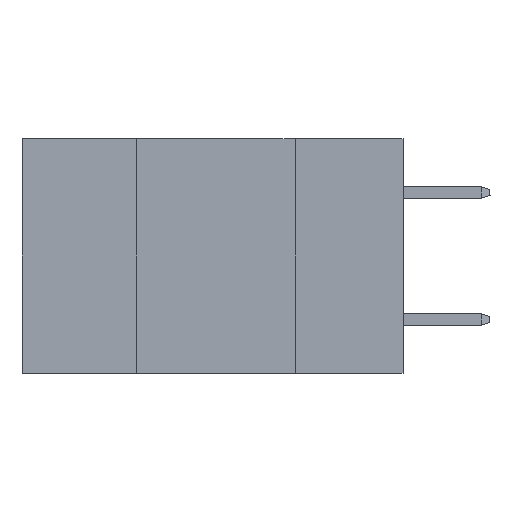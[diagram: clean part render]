
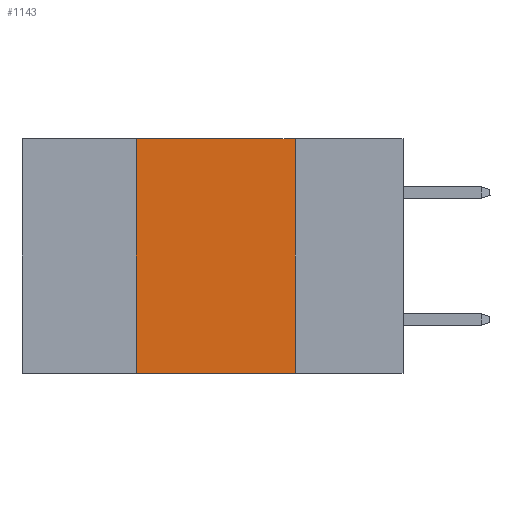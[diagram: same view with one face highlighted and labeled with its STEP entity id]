
A CAD part, left-side view. The second image highlights one B-rep face of the part: STEP entity #1143.
In plain terms, the highlighted planar face has unit normal (-1, 0, 0).
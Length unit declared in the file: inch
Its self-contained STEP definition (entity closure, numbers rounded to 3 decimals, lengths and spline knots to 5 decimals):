
#374 = VERTEX_POINT ( 'NONE', #19718 ) ;
#496 = CARTESIAN_POINT ( 'NONE',  ( 0., 0.17, 0. ) ) ;
#780 = LINE ( 'NONE', #14381, #11953 ) ;
#810 = LINE ( 'NONE', #7644, #19834 ) ;
#1143 = ADVANCED_FACE ( 'NONE', ( #3418 ), #10226, .F. ) ;
#1242 = LINE ( 'NONE', #496, #16465 ) ;
#2068 = DIRECTION ( 'NONE',  ( 1., 0., 0. ) ) ;
#2464 = DIRECTION ( 'NONE',  ( 0., -1., 0. ) ) ;
#3418 = FACE_OUTER_BOUND ( 'NONE', #9105, .T. ) ;
#4226 = LINE ( 'NONE', #11028, #18694 ) ;
#4241 = VERTEX_POINT ( 'NONE', #17039 ) ;
#4633 = ORIENTED_EDGE ( 'NONE', *, *, #12158, .F. ) ;
#6167 = DIRECTION ( 'NONE',  ( 0., 0., -1. ) ) ;
#6919 = ORIENTED_EDGE ( 'NONE', *, *, #18638, .F. ) ;
#7644 = CARTESIAN_POINT ( 'NONE',  ( 0., 0.42, 0. ) ) ;
#9105 = EDGE_LOOP ( 'NONE', ( #10195, #4633, #6919, #14929 ) ) ;
#9787 = EDGE_CURVE ( 'NONE', #374, #21879, #1242, .T. ) ;
#10195 = ORIENTED_EDGE ( 'NONE', *, *, #9787, .F. ) ;
#10226 = PLANE ( 'NONE',  #11723 ) ;
#11028 = CARTESIAN_POINT ( 'NONE',  ( 0., 0.6, 0. ) ) ;
#11723 = AXIS2_PLACEMENT_3D ( 'NONE', #16990, #2068, #12549 ) ;
#11953 = VECTOR ( 'NONE', #2464, 39.37008 ) ;
#12005 = CARTESIAN_POINT ( 'NONE',  ( 0., 0.42, 0. ) ) ;
#12158 = EDGE_CURVE ( 'NONE', #12484, #374, #4226, .T. ) ;
#12484 = VERTEX_POINT ( 'NONE', #12005 ) ;
#12549 = DIRECTION ( 'NONE',  ( 0., 0., -1. ) ) ;
#14363 = DIRECTION ( 'NONE',  ( 0., -1., 0. ) ) ;
#14381 = CARTESIAN_POINT ( 'NONE',  ( 0., 0.6, -0.37 ) ) ;
#14408 = DIRECTION ( 'NONE',  ( 0., 0., 1. ) ) ;
#14929 = ORIENTED_EDGE ( 'NONE', *, *, #17237, .T. ) ;
#16465 = VECTOR ( 'NONE', #6167, 39.37008 ) ;
#16990 = CARTESIAN_POINT ( 'NONE',  ( 0., 0.6, 0. ) ) ;
#17039 = CARTESIAN_POINT ( 'NONE',  ( 0., 0.42, -0.37 ) ) ;
#17237 = EDGE_CURVE ( 'NONE', #4241, #21879, #780, .T. ) ;
#18638 = EDGE_CURVE ( 'NONE', #4241, #12484, #810, .T. ) ;
#18694 = VECTOR ( 'NONE', #14363, 39.37008 ) ;
#19718 = CARTESIAN_POINT ( 'NONE',  ( 0., 0.17, 0. ) ) ;
#19834 = VECTOR ( 'NONE', #14408, 39.37008 ) ;
#21405 = CARTESIAN_POINT ( 'NONE',  ( 0., 0.17, -0.37 ) ) ;
#21879 = VERTEX_POINT ( 'NONE', #21405 ) ;
